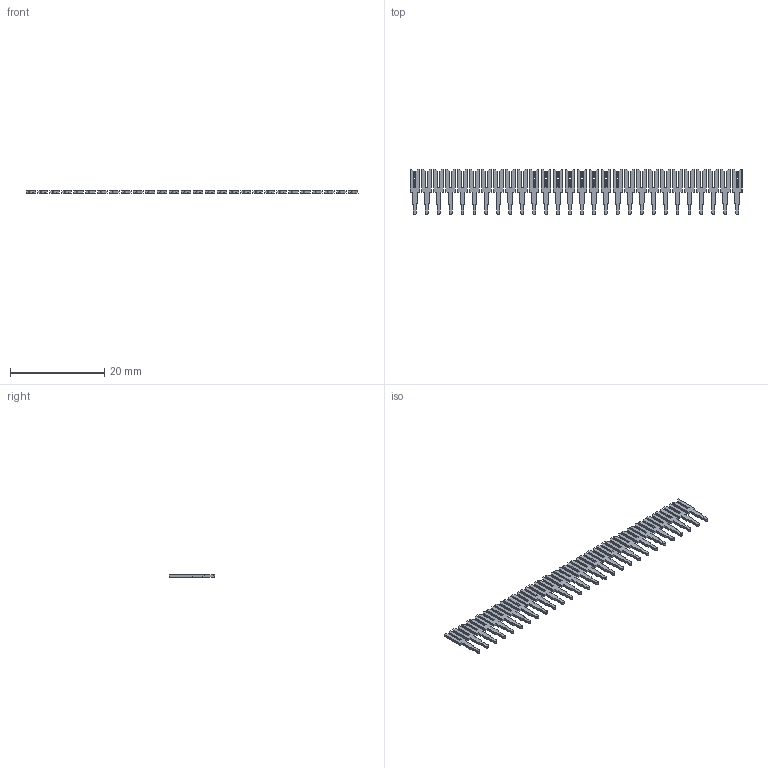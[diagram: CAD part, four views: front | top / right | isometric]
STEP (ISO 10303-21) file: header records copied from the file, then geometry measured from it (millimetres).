
FILE_DESCRIPTION (( 'STEP AP203' ), '1' );
FILE_NAME ('103-028-252-100.STEP', '2020-04-16T15:54:48', ( '' ), ( '' ), 'SwSTEP 2.0', 'SolidWorks 2016', '' );
FILE_SCHEMA (( 'CONFIG_CONTROL_DESIGN' ));
Length unit declared in the file: inch
Products named in the file (2): 103-028-252-100; 100-290-001_100-290-252
Assembly tree (28 placements, depth 2):
  103-028-252-100
    100-290-001_100-290-252  x28
Bounding box: 70.61 x 9.6 x 0.51 mm (x, y, z)
Volume: 171.4 mm3; surface area: 1084.9 mm2
Topology: 28 solids, 28 shells, 672 faces, 1848 edges, 1232 vertices
Faces by surface type: plane 588, cylinder 84
Entity records: 1820 total; most frequent: DIRECTION 182, CARTESIAN_POINT 165, ORIENTED_EDGE 132, CALENDAR_DATE 66, EDGE_CURVE 66, LOCAL_TIME 66, COORDINATED_UNIVERSAL_TIME_OFFSET 66, DATE_AND_TIME 66
